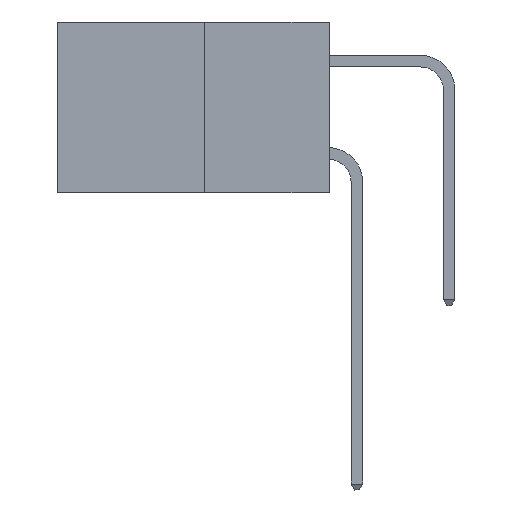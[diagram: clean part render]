
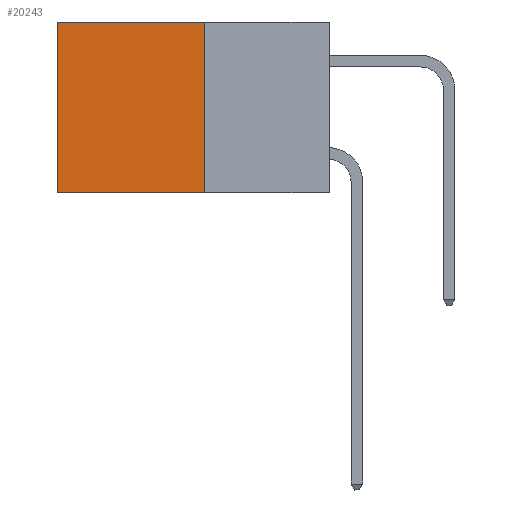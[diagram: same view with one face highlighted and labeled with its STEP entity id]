
A CAD part, left-side view. The second image highlights one B-rep face of the part: STEP entity #20243.
In plain terms, the highlighted planar face has unit normal (-1, 0, 0).
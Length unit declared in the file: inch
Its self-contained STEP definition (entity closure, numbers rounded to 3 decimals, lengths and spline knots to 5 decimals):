
#1424 = VECTOR ( 'NONE', #16605, 39.37008 ) ;
#2740 = EDGE_CURVE ( 'NONE', #7719, #27260, #13024, .T. ) ;
#4199 = EDGE_CURVE ( 'NONE', #27260, #24892, #27576, .T. ) ;
#4679 = CARTESIAN_POINT ( 'NONE',  ( 0.277, 0.27, -0.37 ) ) ;
#4838 = DIRECTION ( 'NONE',  ( 0., 1., 0. ) ) ;
#6483 = EDGE_CURVE ( 'NONE', #7719, #20038, #24432, .T. ) ;
#7719 = VERTEX_POINT ( 'NONE', #22053 ) ;
#9138 = AXIS2_PLACEMENT_3D ( 'NONE', #23174, #12641, #27456 ) ;
#9603 = DIRECTION ( 'NONE',  ( 0., 1., 0. ) ) ;
#10347 = VECTOR ( 'NONE', #22138, 39.37008 ) ;
#12641 = DIRECTION ( 'NONE',  ( 1., 0., 0. ) ) ;
#12885 = FACE_OUTER_BOUND ( 'NONE', #16983, .T. ) ;
#13024 = LINE ( 'NONE', #16660, #1424 ) ;
#16071 = ORIENTED_EDGE ( 'NONE', *, *, #24492, .T. ) ;
#16090 = ORIENTED_EDGE ( 'NONE', *, *, #2740, .F. ) ;
#16605 = DIRECTION ( 'NONE',  ( 0., 0., -1. ) ) ;
#16660 = CARTESIAN_POINT ( 'NONE',  ( 0.277, 0.27, -0.37 ) ) ;
#16983 = EDGE_LOOP ( 'NONE', ( #16071, #24115, #16090, #24455 ) ) ;
#18155 = VECTOR ( 'NONE', #9603, 39.37008 ) ;
#18370 = CARTESIAN_POINT ( 'NONE',  ( 0.277, 0.59, 0. ) ) ;
#19334 = CARTESIAN_POINT ( 'NONE',  ( 0.277, 0.27, 0. ) ) ;
#20001 = CARTESIAN_POINT ( 'NONE',  ( 0.277, 0.59, -0.37 ) ) ;
#20038 = VERTEX_POINT ( 'NONE', #18370 ) ;
#20243 = ADVANCED_FACE ( 'NONE', ( #12885 ), #25318, .F. ) ;
#21695 = CARTESIAN_POINT ( 'NONE',  ( 0.277, 0.27, -0.37 ) ) ;
#21905 = VECTOR ( 'NONE', #4838, 39.37008 ) ;
#22053 = CARTESIAN_POINT ( 'NONE',  ( 0.277, 0.27, 0. ) ) ;
#22138 = DIRECTION ( 'NONE',  ( 0., 0., -1. ) ) ;
#23174 = CARTESIAN_POINT ( 'NONE',  ( 0.277, 0.27, -0.37 ) ) ;
#24115 = ORIENTED_EDGE ( 'NONE', *, *, #4199, .F. ) ;
#24432 = LINE ( 'NONE', #19334, #18155 ) ;
#24455 = ORIENTED_EDGE ( 'NONE', *, *, #6483, .T. ) ;
#24492 = EDGE_CURVE ( 'NONE', #20038, #24892, #27243, .T. ) ;
#24892 = VERTEX_POINT ( 'NONE', #27624 ) ;
#25318 = PLANE ( 'NONE',  #9138 ) ;
#27243 = LINE ( 'NONE', #20001, #10347 ) ;
#27260 = VERTEX_POINT ( 'NONE', #21695 ) ;
#27456 = DIRECTION ( 'NONE',  ( 0., 0., -1. ) ) ;
#27576 = LINE ( 'NONE', #4679, #21905 ) ;
#27624 = CARTESIAN_POINT ( 'NONE',  ( 0.277, 0.59, -0.37 ) ) ;
